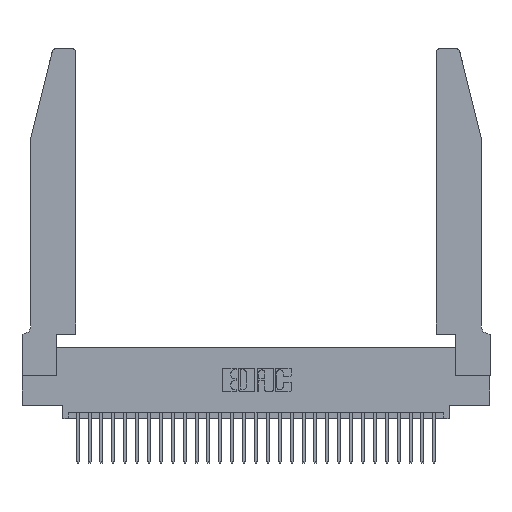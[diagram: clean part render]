
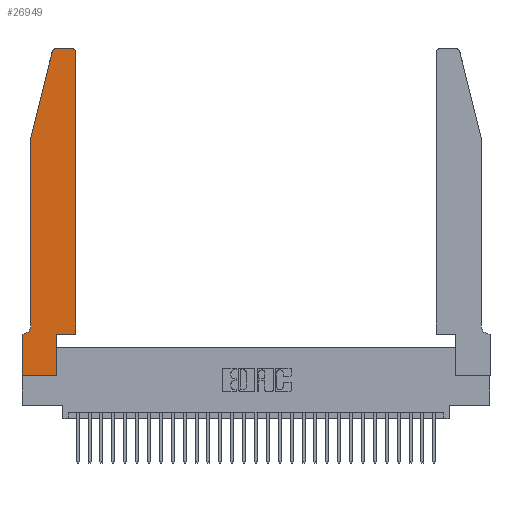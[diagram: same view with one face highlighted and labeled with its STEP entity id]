
A CAD part, top view. The second image highlights one B-rep face of the part: STEP entity #26949.
In plain terms, the highlighted planar face has unit normal (0, 0, 1).
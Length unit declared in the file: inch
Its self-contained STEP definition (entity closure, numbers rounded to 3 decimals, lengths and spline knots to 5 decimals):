
#65 = EDGE_CURVE ( 'NONE', #18852, #16305, #3452, .T. ) ;
#479 = CARTESIAN_POINT ( 'NONE',  ( 0.4505, 0.35, 0.37 ) ) ;
#575 = LINE ( 'NONE', #25527, #27748 ) ;
#634 = CARTESIAN_POINT ( 'NONE',  ( 0., 0., 0.37 ) ) ;
#774 = DIRECTION ( 'NONE',  ( 0., 1., 0. ) ) ;
#1350 = ORIENTED_EDGE ( 'NONE', *, *, #14089, .T. ) ;
#1828 = DIRECTION ( 'NONE',  ( 0., 0., 1. ) ) ;
#1851 = DIRECTION ( 'NONE',  ( 0., 0., 1. ) ) ;
#2300 = VECTOR ( 'NONE', #23507, 39.37008 ) ;
#2569 = VERTEX_POINT ( 'NONE', #22545 ) ;
#2650 = AXIS2_PLACEMENT_3D ( 'NONE', #14079, #28171, #13984 ) ;
#3152 = LINE ( 'NONE', #9492, #3921 ) ;
#3452 = CIRCLE ( 'NONE', #10177, 0.03 ) ;
#3921 = VECTOR ( 'NONE', #9877, 39.37008 ) ;
#4116 = LINE ( 'NONE', #24000, #12282 ) ;
#4448 = DIRECTION ( 'NONE',  ( 1., 0., 0. ) ) ;
#4576 = CARTESIAN_POINT ( 'NONE',  ( 0.2865, 0.35, 0.37 ) ) ;
#4720 = CARTESIAN_POINT ( 'NONE',  ( 0.4505, 0.35, 0.37 ) ) ;
#4979 = EDGE_CURVE ( 'NONE', #10621, #25529, #20751, .T. ) ;
#5151 = VECTOR ( 'NONE', #8922, 39.37008 ) ;
#5332 = CARTESIAN_POINT ( 'NONE',  ( 0., 0.35, 0.37 ) ) ;
#5408 = EDGE_CURVE ( 'NONE', #25529, #29613, #3152, .T. ) ;
#6897 = CARTESIAN_POINT ( 'NONE',  ( 0., 0.35, 0.37 ) ) ;
#7120 = ORIENTED_EDGE ( 'NONE', *, *, #4979, .T. ) ;
#7473 = ORIENTED_EDGE ( 'NONE', *, *, #19466, .T. ) ;
#8922 = DIRECTION ( 'NONE',  ( 0., -1., 0. ) ) ;
#9371 = VERTEX_POINT ( 'NONE', #479 ) ;
#9492 = CARTESIAN_POINT ( 'NONE',  ( 0., 0., 0.37 ) ) ;
#9877 = DIRECTION ( 'NONE',  ( 1., 0., 0. ) ) ;
#10085 = EDGE_CURVE ( 'NONE', #24864, #10621, #575, .T. ) ;
#10177 = AXIS2_PLACEMENT_3D ( 'NONE', #23436, #1851, #4448 ) ;
#10621 = VERTEX_POINT ( 'NONE', #5332 ) ;
#10827 = ORIENTED_EDGE ( 'NONE', *, *, #65, .T. ) ;
#10830 = AXIS2_PLACEMENT_3D ( 'NONE', #6897, #1828, #20816 ) ;
#10970 = ORIENTED_EDGE ( 'NONE', *, *, #23964, .T. ) ;
#11166 = DIRECTION ( 'NONE',  ( -1., 0., 0. ) ) ;
#11349 = CIRCLE ( 'NONE', #2650, 0.07 ) ;
#12064 = CARTESIAN_POINT ( 'NONE',  ( 0.0755, 0.42, 0.37 ) ) ;
#12282 = VECTOR ( 'NONE', #19628, 39.37008 ) ;
#12348 = CIRCLE ( 'NONE', #27176, 0.03 ) ;
#12667 = EDGE_LOOP ( 'NONE', ( #1350, #27556, #20753, #20040, #23131, #28345, #7120, #26933, #27413, #10970, #7473, #10827 ) ) ;
#12759 = LINE ( 'NONE', #29238, #17228 ) ;
#12908 = LINE ( 'NONE', #17687, #21144 ) ;
#13609 = CARTESIAN_POINT ( 'NONE',  ( 0.284, 2.72, 0.37 ) ) ;
#13984 = DIRECTION ( 'NONE',  ( -1., 0., 0. ) ) ;
#14079 = CARTESIAN_POINT ( 'NONE',  ( 0.0055, 0.42, 0.37 ) ) ;
#14089 = EDGE_CURVE ( 'NONE', #16305, #2569, #4116, .T. ) ;
#14955 = CARTESIAN_POINT ( 'NONE',  ( 0.0055, 0.35, 0.37 ) ) ;
#15268 = DIRECTION ( 'NONE',  ( -0.239, -0.971, 0. ) ) ;
#15490 = VERTEX_POINT ( 'NONE', #4576 ) ;
#15664 = LINE ( 'NONE', #23726, #24575 ) ;
#15905 = DIRECTION ( 'NONE',  ( 1., 0., 0. ) ) ;
#16305 = VERTEX_POINT ( 'NONE', #22258 ) ;
#17228 = VECTOR ( 'NONE', #15268, 39.37008 ) ;
#17687 = CARTESIAN_POINT ( 'NONE',  ( 0.2865, 0.35, 0.37 ) ) ;
#18787 = VERTEX_POINT ( 'NONE', #23633 ) ;
#18852 = VERTEX_POINT ( 'NONE', #30410 ) ;
#19289 = EDGE_CURVE ( 'NONE', #2569, #28819, #12348, .T. ) ;
#19466 = EDGE_CURVE ( 'NONE', #9371, #18852, #23903, .T. ) ;
#19628 = DIRECTION ( 'NONE',  ( -1., 0., 0. ) ) ;
#20040 = ORIENTED_EDGE ( 'NONE', *, *, #20642, .T. ) ;
#20145 = VERTEX_POINT ( 'NONE', #12064 ) ;
#20642 = EDGE_CURVE ( 'NONE', #18787, #20145, #28237, .T. ) ;
#20723 = DIRECTION ( 'NONE',  ( 0., 0., 1. ) ) ;
#20751 = LINE ( 'NONE', #634, #30320 ) ;
#20753 = ORIENTED_EDGE ( 'NONE', *, *, #28914, .T. ) ;
#20816 = DIRECTION ( 'NONE',  ( 1., 0., 0. ) ) ;
#21144 = VECTOR ( 'NONE', #774, 39.37008 ) ;
#22254 = CARTESIAN_POINT ( 'NONE',  ( 0.25487, 2.72718, 0.37 ) ) ;
#22258 = CARTESIAN_POINT ( 'NONE',  ( 0.4205, 2.75, 0.37 ) ) ;
#22545 = CARTESIAN_POINT ( 'NONE',  ( 0.284, 2.75, 0.37 ) ) ;
#23131 = ORIENTED_EDGE ( 'NONE', *, *, #28083, .T. ) ;
#23436 = CARTESIAN_POINT ( 'NONE',  ( 0.4205, 2.72, 0.37 ) ) ;
#23507 = DIRECTION ( 'NONE',  ( 0., 1., 0. ) ) ;
#23633 = CARTESIAN_POINT ( 'NONE',  ( 0.0755, 2., 0.37 ) ) ;
#23726 = CARTESIAN_POINT ( 'NONE',  ( 0.4505, 0.35, 0.37 ) ) ;
#23903 = LINE ( 'NONE', #4720, #2300 ) ;
#23964 = EDGE_CURVE ( 'NONE', #15490, #9371, #15664, .T. ) ;
#24000 = CARTESIAN_POINT ( 'NONE',  ( 0.2605, 2.75, 0.37 ) ) ;
#24575 = VECTOR ( 'NONE', #26175, 39.37008 ) ;
#24864 = VERTEX_POINT ( 'NONE', #14955 ) ;
#25316 = CARTESIAN_POINT ( 'NONE',  ( 0.2865, 0., 0.37 ) ) ;
#25527 = CARTESIAN_POINT ( 'NONE',  ( 0.0755, 0.35, 0.37 ) ) ;
#25529 = VERTEX_POINT ( 'NONE', #29843 ) ;
#25689 = CARTESIAN_POINT ( 'NONE',  ( 0.0755, 2., 0.37 ) ) ;
#26175 = DIRECTION ( 'NONE',  ( 1., 0., 0. ) ) ;
#26615 = EDGE_CURVE ( 'NONE', #29613, #15490, #12908, .T. ) ;
#26933 = ORIENTED_EDGE ( 'NONE', *, *, #5408, .T. ) ;
#26949 = ADVANCED_FACE ( 'NONE', ( #26993 ), #28214, .T. ) ;
#26993 = FACE_OUTER_BOUND ( 'NONE', #12667, .T. ) ;
#27176 = AXIS2_PLACEMENT_3D ( 'NONE', #13609, #20723, #15905 ) ;
#27413 = ORIENTED_EDGE ( 'NONE', *, *, #26615, .T. ) ;
#27556 = ORIENTED_EDGE ( 'NONE', *, *, #19289, .T. ) ;
#27748 = VECTOR ( 'NONE', #11166, 39.37008 ) ;
#28083 = EDGE_CURVE ( 'NONE', #20145, #24864, #11349, .T. ) ;
#28171 = DIRECTION ( 'NONE',  ( 0., 0., -1. ) ) ;
#28214 = PLANE ( 'NONE',  #10830 ) ;
#28237 = LINE ( 'NONE', #25689, #5151 ) ;
#28345 = ORIENTED_EDGE ( 'NONE', *, *, #10085, .T. ) ;
#28819 = VERTEX_POINT ( 'NONE', #22254 ) ;
#28914 = EDGE_CURVE ( 'NONE', #28819, #18787, #12759, .T. ) ;
#29238 = CARTESIAN_POINT ( 'NONE',  ( 0.0755, 2., 0.37 ) ) ;
#29423 = DIRECTION ( 'NONE',  ( 0., -1., 0. ) ) ;
#29613 = VERTEX_POINT ( 'NONE', #25316 ) ;
#29843 = CARTESIAN_POINT ( 'NONE',  ( 0., 0., 0.37 ) ) ;
#30320 = VECTOR ( 'NONE', #29423, 39.37008 ) ;
#30410 = CARTESIAN_POINT ( 'NONE',  ( 0.4505, 2.72, 0.37 ) ) ;
